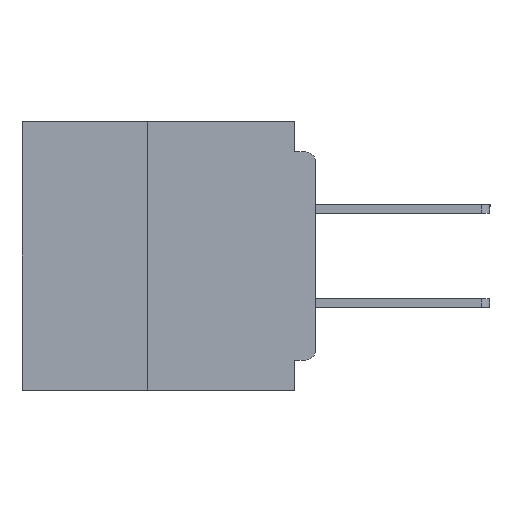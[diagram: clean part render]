
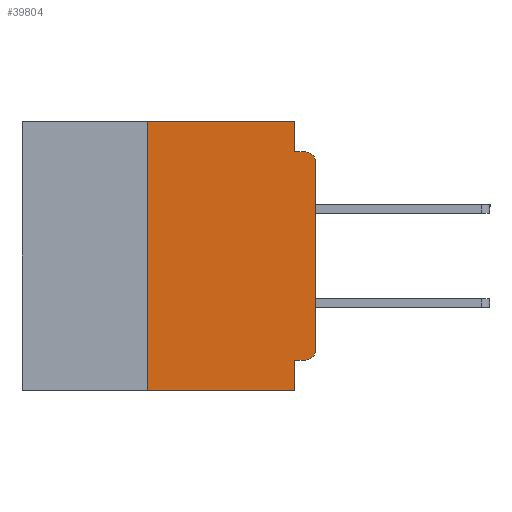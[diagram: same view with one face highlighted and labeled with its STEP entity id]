
A CAD part, left-side view. The second image highlights one B-rep face of the part: STEP entity #39804.
In plain terms, the highlighted planar face has unit normal (-1, 0, 0).
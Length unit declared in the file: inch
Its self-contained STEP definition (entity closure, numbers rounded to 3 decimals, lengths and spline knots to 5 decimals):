
#23 = EDGE_CURVE ( 'NONE', #39134, #3535, #8439, .T. ) ;
#91 = LINE ( 'NONE', #39612, #25810 ) ;
#155 = CARTESIAN_POINT ( 'NONE',  ( 0., 0.031, -0.4 ) ) ;
#264 = CARTESIAN_POINT ( 'NONE',  ( 0., 0., 0. ) ) ;
#591 = ORIENTED_EDGE ( 'NONE', *, *, #42031, .F. ) ;
#1102 = DIRECTION ( 'NONE',  ( 0., 0., -1. ) ) ;
#1456 = LINE ( 'NONE', #26351, #36111 ) ;
#1854 = AXIS2_PLACEMENT_3D ( 'NONE', #24767, #4660, #28179 ) ;
#2646 = EDGE_CURVE ( 'NONE', #37130, #11582, #26717, .T. ) ;
#2911 = EDGE_CURVE ( 'NONE', #3535, #37130, #32960, .T. ) ;
#3535 = VERTEX_POINT ( 'NONE', #25364 ) ;
#3975 = EDGE_CURVE ( 'NONE', #20889, #11582, #27646, .T. ) ;
#4143 = DIRECTION ( 'NONE',  ( 0., -1., 0. ) ) ;
#4660 = DIRECTION ( 'NONE',  ( -1., 0., 0. ) ) ;
#5731 = CARTESIAN_POINT ( 'NONE',  ( 0., 0., -0.06 ) ) ;
#6196 = DIRECTION ( 'NONE',  ( 0., 0., 1. ) ) ;
#7584 = CARTESIAN_POINT ( 'NONE',  ( 0., 0.031, -0.045 ) ) ;
#8439 = LINE ( 'NONE', #36321, #34215 ) ;
#8533 = CARTESIAN_POINT ( 'NONE',  ( 0., 0., -0.355 ) ) ;
#9140 = VERTEX_POINT ( 'NONE', #155 ) ;
#9796 = VERTEX_POINT ( 'NONE', #24308 ) ;
#10097 = CARTESIAN_POINT ( 'NONE',  ( 0., 0.015, -0.355 ) ) ;
#11066 = LINE ( 'NONE', #8533, #27945 ) ;
#11582 = VERTEX_POINT ( 'NONE', #22061 ) ;
#11900 = DIRECTION ( 'NONE',  ( 0., 1., 0. ) ) ;
#11946 = ORIENTED_EDGE ( 'NONE', *, *, #23, .F. ) ;
#12161 = DIRECTION ( 'NONE',  ( 0., 0., -1. ) ) ;
#12348 = LINE ( 'NONE', #29493, #29237 ) ;
#12849 = LINE ( 'NONE', #264, #21788 ) ;
#14260 = VERTEX_POINT ( 'NONE', #16904 ) ;
#14622 = CARTESIAN_POINT ( 'NONE',  ( 0., 0.25, 0. ) ) ;
#15099 = EDGE_CURVE ( 'NONE', #27368, #41521, #39137, .T. ) ;
#15499 = ORIENTED_EDGE ( 'NONE', *, *, #2646, .F. ) ;
#16086 = DIRECTION ( 'NONE',  ( 0., 0., -1. ) ) ;
#16904 = CARTESIAN_POINT ( 'NONE',  ( 0., 0.031, -0.355 ) ) ;
#17681 = DIRECTION ( 'NONE',  ( 0., -1., 0. ) ) ;
#17759 = VECTOR ( 'NONE', #4143, 39.37008 ) ;
#19741 = ORIENTED_EDGE ( 'NONE', *, *, #39411, .F. ) ;
#19758 = DIRECTION ( 'NONE',  ( 0., 0., -1. ) ) ;
#20237 = ORIENTED_EDGE ( 'NONE', *, *, #21714, .T. ) ;
#20889 = VERTEX_POINT ( 'NONE', #5731 ) ;
#21209 = DIRECTION ( 'NONE',  ( -1., 0., 0. ) ) ;
#21714 = EDGE_CURVE ( 'NONE', #41521, #20889, #12849, .T. ) ;
#21788 = VECTOR ( 'NONE', #37212, 39.37008 ) ;
#22061 = CARTESIAN_POINT ( 'NONE',  ( 0., 0.015, -0.045 ) ) ;
#22992 = CARTESIAN_POINT ( 'NONE',  ( 0., 0.437, 0. ) ) ;
#24308 = CARTESIAN_POINT ( 'NONE',  ( 0., 0.25, -0.4 ) ) ;
#24767 = CARTESIAN_POINT ( 'NONE',  ( 0., 0.015, -0.34 ) ) ;
#25364 = CARTESIAN_POINT ( 'NONE',  ( 0., 0.031, 0. ) ) ;
#25810 = VECTOR ( 'NONE', #29583, 39.37008 ) ;
#26351 = CARTESIAN_POINT ( 'NONE',  ( 0., 0.25, -0.4 ) ) ;
#26717 = LINE ( 'NONE', #30742, #17759 ) ;
#27368 = VERTEX_POINT ( 'NONE', #10097 ) ;
#27646 = CIRCLE ( 'NONE', #41072, 0.015 ) ;
#27945 = VECTOR ( 'NONE', #11900, 39.37008 ) ;
#27985 = AXIS2_PLACEMENT_3D ( 'NONE', #22992, #39812, #19758 ) ;
#28179 = DIRECTION ( 'NONE',  ( 0., 0., -1. ) ) ;
#29237 = VECTOR ( 'NONE', #16086, 39.37008 ) ;
#29493 = CARTESIAN_POINT ( 'NONE',  ( 0., 0.031, -0.4 ) ) ;
#29583 = DIRECTION ( 'NONE',  ( 0., -1., 0. ) ) ;
#29760 = PLANE ( 'NONE',  #27985 ) ;
#30446 = EDGE_CURVE ( 'NONE', #9796, #9140, #91, .T. ) ;
#30742 = CARTESIAN_POINT ( 'NONE',  ( 0., 0., -0.045 ) ) ;
#31335 = ORIENTED_EDGE ( 'NONE', *, *, #30446, .T. ) ;
#31405 = ORIENTED_EDGE ( 'NONE', *, *, #15099, .T. ) ;
#32960 = LINE ( 'NONE', #35665, #40780 ) ;
#34215 = VECTOR ( 'NONE', #17681, 39.37008 ) ;
#35665 = CARTESIAN_POINT ( 'NONE',  ( 0., 0.031, 0. ) ) ;
#35666 = ORIENTED_EDGE ( 'NONE', *, *, #2911, .F. ) ;
#36032 = CARTESIAN_POINT ( 'NONE',  ( 0., 0., -0.34 ) ) ;
#36111 = VECTOR ( 'NONE', #6196, 39.37008 ) ;
#36321 = CARTESIAN_POINT ( 'NONE',  ( 0., 0.437, 0. ) ) ;
#37130 = VERTEX_POINT ( 'NONE', #7584 ) ;
#37212 = DIRECTION ( 'NONE',  ( 0., 0., 1. ) ) ;
#37490 = ORIENTED_EDGE ( 'NONE', *, *, #38150, .F. ) ;
#38150 = EDGE_CURVE ( 'NONE', #9796, #39134, #1456, .T. ) ;
#39074 = FACE_OUTER_BOUND ( 'NONE', #40439, .T. ) ;
#39134 = VERTEX_POINT ( 'NONE', #14622 ) ;
#39137 = CIRCLE ( 'NONE', #1854, 0.015 ) ;
#39411 = EDGE_CURVE ( 'NONE', #14260, #9140, #12348, .T. ) ;
#39612 = CARTESIAN_POINT ( 'NONE',  ( 0., 0.437, -0.4 ) ) ;
#39804 = ADVANCED_FACE ( 'NONE', ( #39074 ), #29760, .F. ) ;
#39812 = DIRECTION ( 'NONE',  ( 1., 0., 0. ) ) ;
#40439 = EDGE_LOOP ( 'NONE', ( #20237, #42480, #15499, #35666, #11946, #37490, #31335, #19741, #591, #31405 ) ) ;
#40780 = VECTOR ( 'NONE', #12161, 39.37008 ) ;
#41072 = AXIS2_PLACEMENT_3D ( 'NONE', #41255, #21209, #1102 ) ;
#41255 = CARTESIAN_POINT ( 'NONE',  ( 0., 0.015, -0.06 ) ) ;
#41521 = VERTEX_POINT ( 'NONE', #36032 ) ;
#42031 = EDGE_CURVE ( 'NONE', #27368, #14260, #11066, .T. ) ;
#42480 = ORIENTED_EDGE ( 'NONE', *, *, #3975, .T. ) ;
